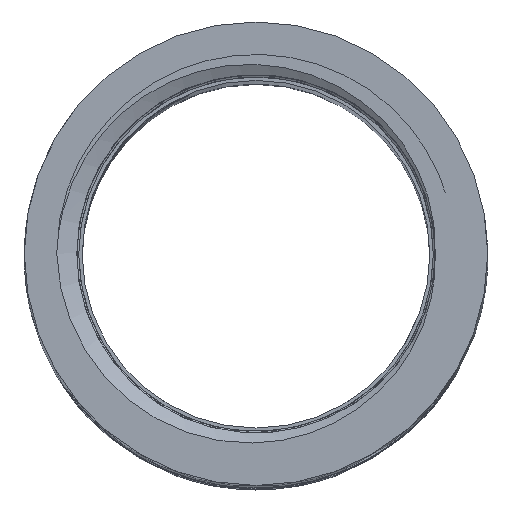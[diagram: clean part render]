
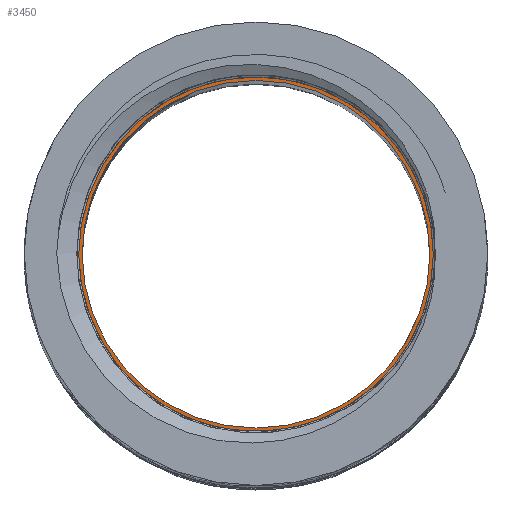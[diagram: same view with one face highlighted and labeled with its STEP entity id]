
A CAD part, top view. The second image highlights one B-rep face of the part: STEP entity #3450.
In plain terms, the highlighted planar face has unit normal (0, 0, 1).
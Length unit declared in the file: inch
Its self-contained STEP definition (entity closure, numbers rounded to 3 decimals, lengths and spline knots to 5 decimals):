
#460 = VERTEX_POINT ( 'NONE', #2587 ) ;
#911 = FACE_BOUND ( 'NONE', #4130, .T. ) ;
#1137 = FACE_OUTER_BOUND ( 'NONE', #5470, .T. ) ;
#1302 = CARTESIAN_POINT ( 'NONE',  ( 0.3825, 0., 5.027 ) ) ;
#1527 = CIRCLE ( 'NONE', #5179, 0.3825 ) ;
#1530 = AXIS2_PLACEMENT_3D ( 'NONE', #7549, #7005, #2645 ) ;
#1690 = DIRECTION ( 'NONE',  ( 0., 0., 1. ) ) ;
#2232 = ORIENTED_EDGE ( 'NONE', *, *, #3030, .F. ) ;
#2378 = AXIS2_PLACEMENT_3D ( 'NONE', #7937, #6687, #3760 ) ;
#2443 = PLANE ( 'NONE',  #1530 ) ;
#2537 = CARTESIAN_POINT ( 'NONE',  ( 0., 0., 5.027 ) ) ;
#2575 = ORIENTED_EDGE ( 'NONE', *, *, #8166, .T. ) ;
#2587 = CARTESIAN_POINT ( 'NONE',  ( -0.375, 0., 5.027 ) ) ;
#2645 = DIRECTION ( 'NONE',  ( 1., 0., 0. ) ) ;
#2761 = CIRCLE ( 'NONE', #7906, 0.375 ) ;
#3030 = EDGE_CURVE ( 'NONE', #7611, #460, #6356, .T. ) ;
#3214 = CIRCLE ( 'NONE', #3454, 0.3825 ) ;
#3450 = ADVANCED_FACE ( 'NONE', ( #911, #1137 ), #2443, .T. ) ;
#3454 = AXIS2_PLACEMENT_3D ( 'NONE', #2537, #4722, #9086 ) ;
#3760 = DIRECTION ( 'NONE',  ( 1., 0., 0. ) ) ;
#4130 = EDGE_LOOP ( 'NONE', ( #5992, #2232 ) ) ;
#4722 = DIRECTION ( 'NONE',  ( 0., 0., 1. ) ) ;
#4816 = CARTESIAN_POINT ( 'NONE',  ( 0., 0., 5.027 ) ) ;
#5179 = AXIS2_PLACEMENT_3D ( 'NONE', #8268, #1690, #6855 ) ;
#5190 = ORIENTED_EDGE ( 'NONE', *, *, #6000, .T. ) ;
#5470 = EDGE_LOOP ( 'NONE', ( #2575, #5190 ) ) ;
#5543 = DIRECTION ( 'NONE',  ( 1., 0., 0. ) ) ;
#5992 = ORIENTED_EDGE ( 'NONE', *, *, #6704, .F. ) ;
#6000 = EDGE_CURVE ( 'NONE', #9317, #7946, #1527, .T. ) ;
#6140 = CARTESIAN_POINT ( 'NONE',  ( 0.375, 0., 5.027 ) ) ;
#6356 = CIRCLE ( 'NONE', #2378, 0.375 ) ;
#6687 = DIRECTION ( 'NONE',  ( 0., 0., 1. ) ) ;
#6704 = EDGE_CURVE ( 'NONE', #460, #7611, #2761, .T. ) ;
#6855 = DIRECTION ( 'NONE',  ( 1., 0., 0. ) ) ;
#7005 = DIRECTION ( 'NONE',  ( 0., 0., 1. ) ) ;
#7549 = CARTESIAN_POINT ( 'NONE',  ( 0., 0., 5.027 ) ) ;
#7611 = VERTEX_POINT ( 'NONE', #6140 ) ;
#7906 = AXIS2_PLACEMENT_3D ( 'NONE', #4816, #9217, #5543 ) ;
#7937 = CARTESIAN_POINT ( 'NONE',  ( 0., 0., 5.027 ) ) ;
#7946 = VERTEX_POINT ( 'NONE', #1302 ) ;
#8166 = EDGE_CURVE ( 'NONE', #7946, #9317, #3214, .T. ) ;
#8268 = CARTESIAN_POINT ( 'NONE',  ( 0., 0., 5.027 ) ) ;
#8992 = CARTESIAN_POINT ( 'NONE',  ( -0.3825, 0., 5.027 ) ) ;
#9086 = DIRECTION ( 'NONE',  ( 1., 0., 0. ) ) ;
#9217 = DIRECTION ( 'NONE',  ( 0., 0., 1. ) ) ;
#9317 = VERTEX_POINT ( 'NONE', #8992 ) ;
